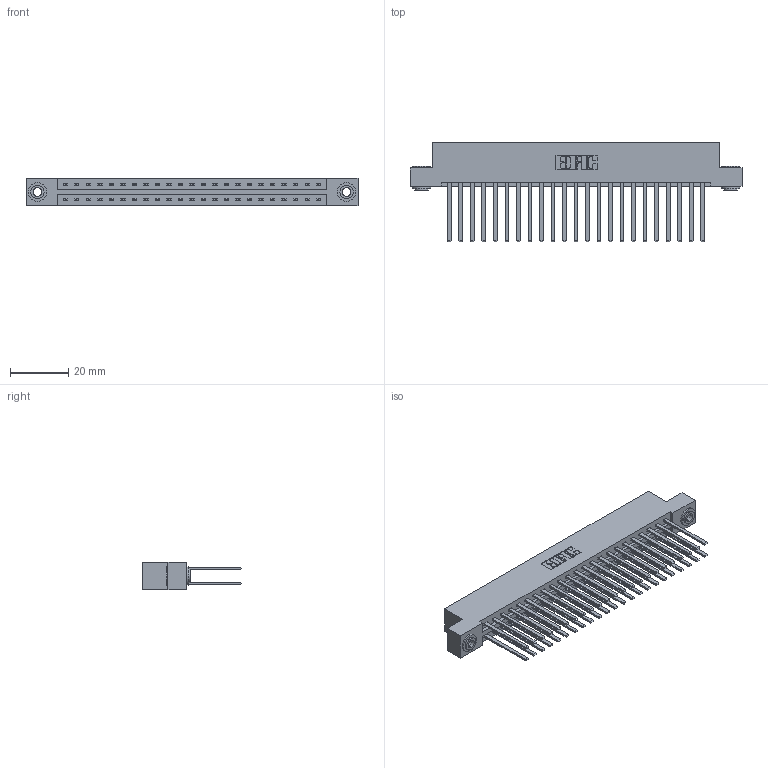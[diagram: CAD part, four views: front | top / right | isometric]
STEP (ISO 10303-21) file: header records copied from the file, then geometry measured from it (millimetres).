
FILE_DESCRIPTION (( 'STEP AP203' ), '1' );
FILE_NAME ('387-046-544-203.STEP', '2018-09-20T04:17:42', ( '' ), ( '' ), 'SwSTEP 2.0', 'SolidWorks 2016', '' );
FILE_SCHEMA (( 'CONFIG_CONTROL_DESIGN' ));
Length unit declared in the file: inch
Products named in the file (4): 337 Part_Flush Mounting Lugs - 0.156 Dia-TH; 345-292-001_345-293-144; 345-250-002_345-250-002-102; 387-046-544-203
Assembly tree (49 placements, depth 2):
  387-046-544-203
    337 Part_Flush Mounting Lugs - 0.156 Dia-TH
    345-292-001_345-293-144  x46
    345-250-002_345-250-002-102  x2
Bounding box: 114.15 x 34.3 x 9.4 mm (x, y, z)
Volume: 12441.1 mm3; surface area: 16211 mm2
Topology: 49 solids, 49 shells, 2360 faces, 6965 edges, 4578 vertices
Faces by surface type: plane 1644, cylinder 708, cone 8
Entity records: 20756 total; most frequent: CARTESIAN_POINT 3485, ORIENTED_EDGE 3414, DIRECTION 3029, EDGE_CURVE 1707, LINE 1559, VECTOR 1559, VERTEX_POINT 1134, AXIS2_PLACEMENT_3D 735
